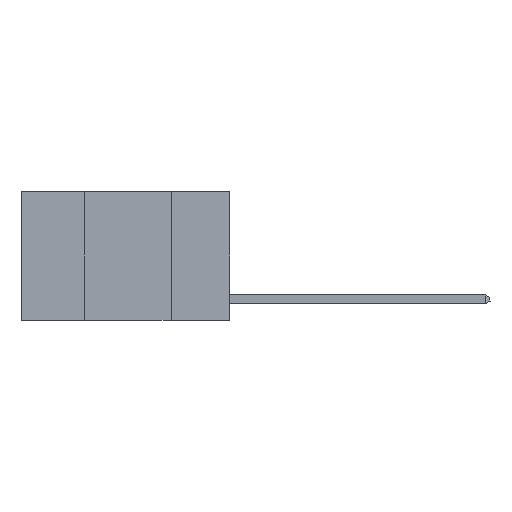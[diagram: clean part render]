
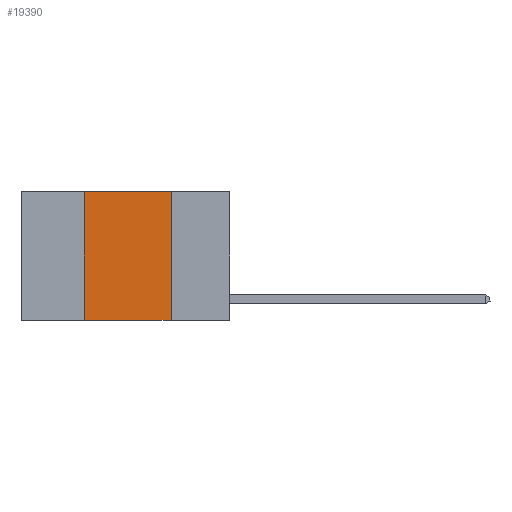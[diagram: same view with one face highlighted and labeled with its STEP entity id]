
A CAD part, left-side view. The second image highlights one B-rep face of the part: STEP entity #19390.
In plain terms, the highlighted planar face has unit normal (-1, 0, 0).
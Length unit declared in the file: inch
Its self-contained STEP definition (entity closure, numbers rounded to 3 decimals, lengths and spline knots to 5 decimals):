
#434 = CARTESIAN_POINT ( 'NONE',  ( 0., 0.17, 0. ) ) ;
#483 = EDGE_CURVE ( 'NONE', #19027, #5063, #6775, .T. ) ;
#1302 = VECTOR ( 'NONE', #8215, 39.37008 ) ;
#1617 = ORIENTED_EDGE ( 'NONE', *, *, #483, .F. ) ;
#1630 = DIRECTION ( 'NONE',  ( 0., -1., 0. ) ) ;
#5063 = VERTEX_POINT ( 'NONE', #22637 ) ;
#5147 = VECTOR ( 'NONE', #11651, 39.37008 ) ;
#5520 = VERTEX_POINT ( 'NONE', #434 ) ;
#5896 = CARTESIAN_POINT ( 'NONE',  ( 0., 0.17, -0.37 ) ) ;
#6775 = LINE ( 'NONE', #8605, #9275 ) ;
#7483 = ORIENTED_EDGE ( 'NONE', *, *, #16291, .F. ) ;
#7743 = VECTOR ( 'NONE', #1630, 39.37008 ) ;
#8215 = DIRECTION ( 'NONE',  ( 0., 0., -1. ) ) ;
#8318 = AXIS2_PLACEMENT_3D ( 'NONE', #25344, #15683, #13453 ) ;
#8502 = LINE ( 'NONE', #17549, #5147 ) ;
#8605 = CARTESIAN_POINT ( 'NONE',  ( 0., 0.42, 0. ) ) ;
#8737 = EDGE_CURVE ( 'NONE', #19027, #17932, #8502, .T. ) ;
#9275 = VECTOR ( 'NONE', #12332, 39.37008 ) ;
#11018 = ORIENTED_EDGE ( 'NONE', *, *, #8737, .T. ) ;
#11271 = CARTESIAN_POINT ( 'NONE',  ( 0., 0.6, 0. ) ) ;
#11547 = PLANE ( 'NONE',  #8318 ) ;
#11651 = DIRECTION ( 'NONE',  ( 0., -1., 0. ) ) ;
#12332 = DIRECTION ( 'NONE',  ( 0., 0., 1. ) ) ;
#13453 = DIRECTION ( 'NONE',  ( 0., 0., -1. ) ) ;
#14596 = ORIENTED_EDGE ( 'NONE', *, *, #19292, .F. ) ;
#15683 = DIRECTION ( 'NONE',  ( 1., 0., 0. ) ) ;
#16080 = CARTESIAN_POINT ( 'NONE',  ( 0., 0.17, 0. ) ) ;
#16291 = EDGE_CURVE ( 'NONE', #5520, #17932, #19533, .T. ) ;
#17078 = FACE_OUTER_BOUND ( 'NONE', #20510, .T. ) ;
#17549 = CARTESIAN_POINT ( 'NONE',  ( 0., 0.6, -0.37 ) ) ;
#17932 = VERTEX_POINT ( 'NONE', #5896 ) ;
#19027 = VERTEX_POINT ( 'NONE', #22542 ) ;
#19292 = EDGE_CURVE ( 'NONE', #5063, #5520, #22225, .T. ) ;
#19390 = ADVANCED_FACE ( 'NONE', ( #17078 ), #11547, .F. ) ;
#19533 = LINE ( 'NONE', #16080, #1302 ) ;
#20510 = EDGE_LOOP ( 'NONE', ( #7483, #14596, #1617, #11018 ) ) ;
#22225 = LINE ( 'NONE', #11271, #7743 ) ;
#22542 = CARTESIAN_POINT ( 'NONE',  ( 0., 0.42, -0.37 ) ) ;
#22637 = CARTESIAN_POINT ( 'NONE',  ( 0., 0.42, 0. ) ) ;
#25344 = CARTESIAN_POINT ( 'NONE',  ( 0., 0.6, 0. ) ) ;
